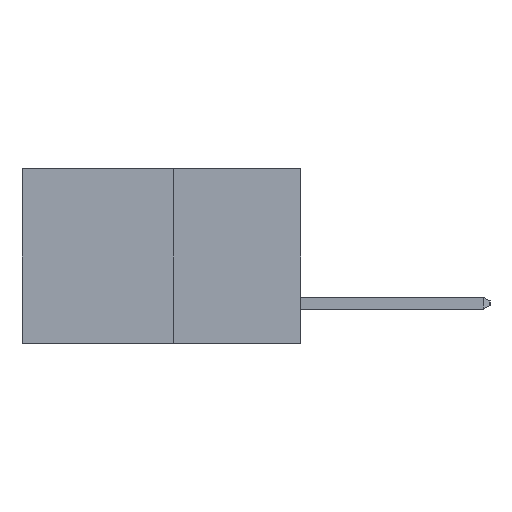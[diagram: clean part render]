
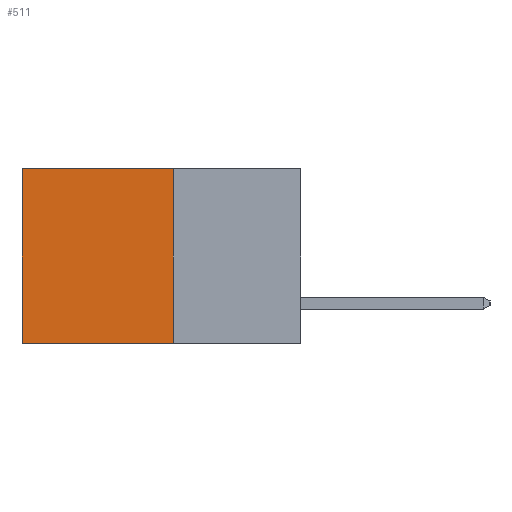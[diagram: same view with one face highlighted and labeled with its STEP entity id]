
A CAD part, left-side view. The second image highlights one B-rep face of the part: STEP entity #511.
In plain terms, the highlighted planar face has unit normal (-1, 0, 0).
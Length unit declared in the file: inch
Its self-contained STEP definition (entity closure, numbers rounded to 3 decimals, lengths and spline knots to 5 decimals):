
#43 = ORIENTED_EDGE ( 'NONE', *, *, #12168, .F. ) ;
#119 = DIRECTION ( 'NONE',  ( 0., 0., -1. ) ) ;
#237 = VERTEX_POINT ( 'NONE', #655 ) ;
#303 = LINE ( 'NONE', #7483, #7986 ) ;
#345 = VECTOR ( 'NONE', #10452, 39.37008 ) ;
#425 = EDGE_CURVE ( 'NONE', #7094, #588, #303, .T. ) ;
#511 = ADVANCED_FACE ( 'NONE', ( #2001 ), #4797, .F. ) ;
#588 = VERTEX_POINT ( 'NONE', #4809 ) ;
#655 = CARTESIAN_POINT ( 'NONE',  ( 0.277, 0.27, 0. ) ) ;
#1567 = DIRECTION ( 'NONE',  ( 0., 0., -1. ) ) ;
#1779 = DIRECTION ( 'NONE',  ( 0., 1., 0. ) ) ;
#1854 = DIRECTION ( 'NONE',  ( 1., 0., 0. ) ) ;
#2001 = FACE_OUTER_BOUND ( 'NONE', #8148, .T. ) ;
#2190 = VECTOR ( 'NONE', #119, 39.37008 ) ;
#2371 = CARTESIAN_POINT ( 'NONE',  ( 0.277, 0.27, -0.37 ) ) ;
#2375 = ORIENTED_EDGE ( 'NONE', *, *, #12511, .F. ) ;
#4408 = CARTESIAN_POINT ( 'NONE',  ( 0.277, 0.27, -0.37 ) ) ;
#4730 = ORIENTED_EDGE ( 'NONE', *, *, #425, .T. ) ;
#4797 = PLANE ( 'NONE',  #10786 ) ;
#4809 = CARTESIAN_POINT ( 'NONE',  ( 0.277, 0.59, -0.37 ) ) ;
#5245 = LINE ( 'NONE', #10580, #7583 ) ;
#6206 = CARTESIAN_POINT ( 'NONE',  ( 0.277, 0.27, -0.37 ) ) ;
#7094 = VERTEX_POINT ( 'NONE', #9876 ) ;
#7483 = CARTESIAN_POINT ( 'NONE',  ( 0.277, 0.59, -0.37 ) ) ;
#7583 = VECTOR ( 'NONE', #1779, 39.37008 ) ;
#7986 = VECTOR ( 'NONE', #1567, 39.37008 ) ;
#8148 = EDGE_LOOP ( 'NONE', ( #4730, #2375, #43, #9907 ) ) ;
#8182 = EDGE_CURVE ( 'NONE', #237, #7094, #5245, .T. ) ;
#9744 = LINE ( 'NONE', #6206, #2190 ) ;
#9876 = CARTESIAN_POINT ( 'NONE',  ( 0.277, 0.59, 0. ) ) ;
#9907 = ORIENTED_EDGE ( 'NONE', *, *, #8182, .T. ) ;
#10287 = VERTEX_POINT ( 'NONE', #4408 ) ;
#10452 = DIRECTION ( 'NONE',  ( 0., 1., 0. ) ) ;
#10579 = LINE ( 'NONE', #12262, #345 ) ;
#10580 = CARTESIAN_POINT ( 'NONE',  ( 0.277, 0.27, 0. ) ) ;
#10786 = AXIS2_PLACEMENT_3D ( 'NONE', #2371, #1854, #11754 ) ;
#11754 = DIRECTION ( 'NONE',  ( 0., 0., -1. ) ) ;
#12168 = EDGE_CURVE ( 'NONE', #237, #10287, #9744, .T. ) ;
#12262 = CARTESIAN_POINT ( 'NONE',  ( 0.277, 0.27, -0.37 ) ) ;
#12511 = EDGE_CURVE ( 'NONE', #10287, #588, #10579, .T. ) ;
